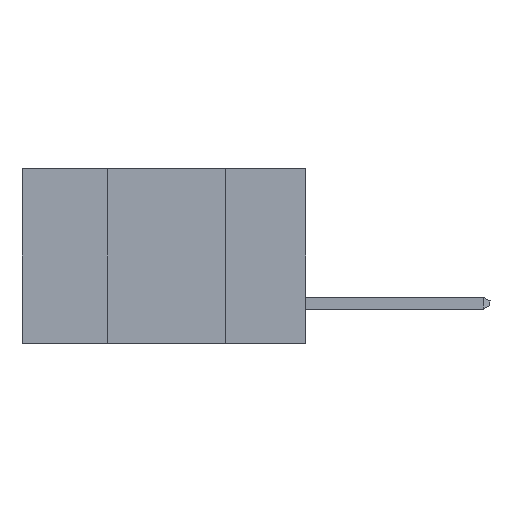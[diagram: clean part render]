
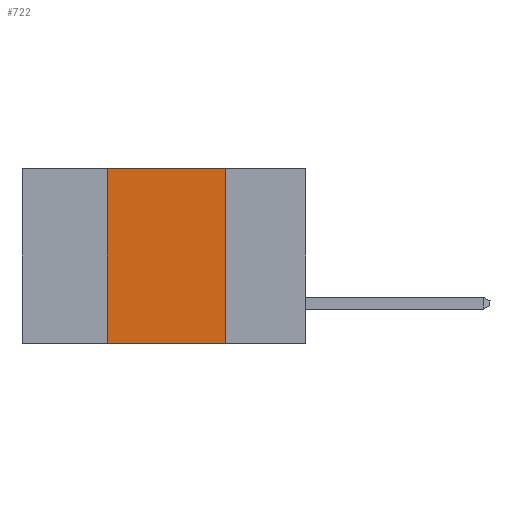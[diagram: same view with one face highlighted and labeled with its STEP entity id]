
A CAD part, left-side view. The second image highlights one B-rep face of the part: STEP entity #722.
In plain terms, the highlighted planar face has unit normal (-1, 0, 0).
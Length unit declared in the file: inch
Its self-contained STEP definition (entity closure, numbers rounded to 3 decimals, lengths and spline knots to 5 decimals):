
#139 = DIRECTION ( 'NONE',  ( 1., 0., 0. ) ) ;
#722 = ADVANCED_FACE ( 'NONE', ( #3275 ), #11412, .F. ) ;
#1248 = CARTESIAN_POINT ( 'NONE',  ( 0., 0.42, 0. ) ) ;
#1423 = LINE ( 'NONE', #4122, #11822 ) ;
#2596 = ORIENTED_EDGE ( 'NONE', *, *, #16480, .F. ) ;
#3275 = FACE_OUTER_BOUND ( 'NONE', #5097, .T. ) ;
#3445 = VERTEX_POINT ( 'NONE', #5463 ) ;
#3858 = DIRECTION ( 'NONE',  ( 0., 0., -1. ) ) ;
#3995 = VECTOR ( 'NONE', #10550, 39.37008 ) ;
#4122 = CARTESIAN_POINT ( 'NONE',  ( 0., 0.6, 0. ) ) ;
#4706 = CARTESIAN_POINT ( 'NONE',  ( 0., 0.6, 0. ) ) ;
#4920 = LINE ( 'NONE', #11718, #16028 ) ;
#5097 = EDGE_LOOP ( 'NONE', ( #2596, #10657, #6642, #9796 ) ) ;
#5463 = CARTESIAN_POINT ( 'NONE',  ( 0., 0.42, -0.37 ) ) ;
#5521 = VERTEX_POINT ( 'NONE', #7722 ) ;
#5843 = DIRECTION ( 'NONE',  ( 0., -1., 0. ) ) ;
#6085 = VERTEX_POINT ( 'NONE', #8357 ) ;
#6489 = EDGE_CURVE ( 'NONE', #15277, #5521, #1423, .T. ) ;
#6642 = ORIENTED_EDGE ( 'NONE', *, *, #9007, .F. ) ;
#6682 = VECTOR ( 'NONE', #5843, 39.37008 ) ;
#7191 = DIRECTION ( 'NONE',  ( 0., 0., -1. ) ) ;
#7722 = CARTESIAN_POINT ( 'NONE',  ( 0., 0.17, 0. ) ) ;
#7744 = DIRECTION ( 'NONE',  ( 0., -1., 0. ) ) ;
#8357 = CARTESIAN_POINT ( 'NONE',  ( 0., 0.17, -0.37 ) ) ;
#9007 = EDGE_CURVE ( 'NONE', #3445, #15277, #13224, .T. ) ;
#9796 = ORIENTED_EDGE ( 'NONE', *, *, #10224, .T. ) ;
#10224 = EDGE_CURVE ( 'NONE', #3445, #6085, #13874, .T. ) ;
#10550 = DIRECTION ( 'NONE',  ( 0., 0., 1. ) ) ;
#10657 = ORIENTED_EDGE ( 'NONE', *, *, #6489, .F. ) ;
#11412 = PLANE ( 'NONE',  #15279 ) ;
#11718 = CARTESIAN_POINT ( 'NONE',  ( 0., 0.17, -0.37 ) ) ;
#11822 = VECTOR ( 'NONE', #7744, 39.37008 ) ;
#13224 = LINE ( 'NONE', #15587, #3995 ) ;
#13874 = LINE ( 'NONE', #15355, #6682 ) ;
#15277 = VERTEX_POINT ( 'NONE', #1248 ) ;
#15279 = AXIS2_PLACEMENT_3D ( 'NONE', #4706, #139, #7191 ) ;
#15355 = CARTESIAN_POINT ( 'NONE',  ( 0., 0.6, -0.37 ) ) ;
#15587 = CARTESIAN_POINT ( 'NONE',  ( 0., 0.42, -0.37 ) ) ;
#16028 = VECTOR ( 'NONE', #3858, 39.37008 ) ;
#16480 = EDGE_CURVE ( 'NONE', #5521, #6085, #4920, .T. ) ;
